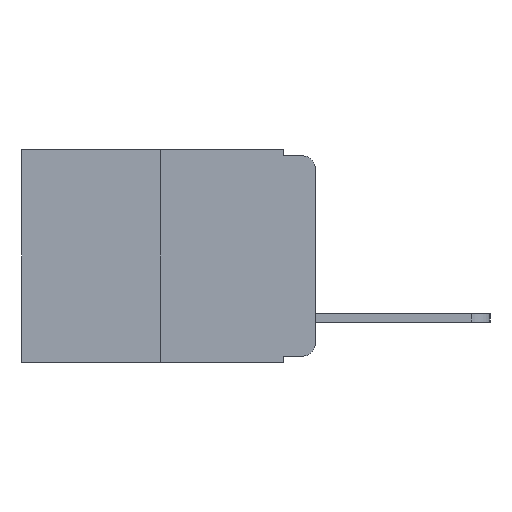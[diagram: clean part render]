
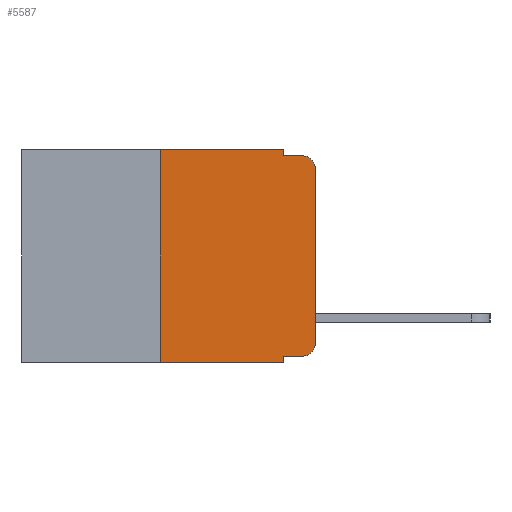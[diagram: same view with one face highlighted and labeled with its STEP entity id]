
A CAD part, left-side view. The second image highlights one B-rep face of the part: STEP entity #5587.
In plain terms, the highlighted planar face has unit normal (-1, 0, 0).
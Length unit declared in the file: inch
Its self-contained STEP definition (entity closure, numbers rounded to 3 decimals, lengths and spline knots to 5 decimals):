
#275 = VERTEX_POINT ( 'NONE', #3671 ) ;
#332 = VERTEX_POINT ( 'NONE', #5225 ) ;
#398 = AXIS2_PLACEMENT_3D ( 'NONE', #10428, #5423, #5416 ) ;
#938 = CARTESIAN_POINT ( 'NONE',  ( 0., 0.25, 0. ) ) ;
#1003 = DIRECTION ( 'NONE',  ( -1., 0., 0. ) ) ;
#1064 = DIRECTION ( 'NONE',  ( -1., 0., 0. ) ) ;
#1121 = DIRECTION ( 'NONE',  ( 0., 0., -1. ) ) ;
#1155 = VERTEX_POINT ( 'NONE', #1823 ) ;
#1223 = VERTEX_POINT ( 'NONE', #1884 ) ;
#1278 = DIRECTION ( 'NONE',  ( 0., 0., 1. ) ) ;
#1470 = CARTESIAN_POINT ( 'NONE',  ( 0., 0.25, 0. ) ) ;
#1720 = EDGE_CURVE ( 'NONE', #7638, #2436, #1954, .T. ) ;
#1823 = CARTESIAN_POINT ( 'NONE',  ( 0., 0.02, -0.01 ) ) ;
#1848 = EDGE_CURVE ( 'NONE', #1223, #10946, #10896, .T. ) ;
#1884 = CARTESIAN_POINT ( 'NONE',  ( 0., 0., -0.313 ) ) ;
#1954 = LINE ( 'NONE', #11174, #9098 ) ;
#2143 = LINE ( 'NONE', #1470, #2428 ) ;
#2428 = VECTOR ( 'NONE', #1278, 39.37008 ) ;
#2436 = VERTEX_POINT ( 'NONE', #6004 ) ;
#2580 = CIRCLE ( 'NONE', #11816, 0.02 ) ;
#2710 = EDGE_CURVE ( 'NONE', #8358, #332, #7228, .T. ) ;
#3127 = VERTEX_POINT ( 'NONE', #7342 ) ;
#3671 = CARTESIAN_POINT ( 'NONE',  ( 0., 0.051, -0.01 ) ) ;
#3939 = CIRCLE ( 'NONE', #5981, 0.02 ) ;
#4093 = EDGE_CURVE ( 'NONE', #3127, #8628, #4499, .T. ) ;
#4331 = LINE ( 'NONE', #4893, #11268 ) ;
#4339 = VECTOR ( 'NONE', #1121, 39.37008 ) ;
#4391 = VECTOR ( 'NONE', #6824, 39.37008 ) ;
#4499 = LINE ( 'NONE', #6081, #11632 ) ;
#4658 = EDGE_CURVE ( 'NONE', #8358, #8628, #6889, .T. ) ;
#4893 = CARTESIAN_POINT ( 'NONE',  ( 0., 0.051, 0. ) ) ;
#5225 = CARTESIAN_POINT ( 'NONE',  ( 0., 0.02, -0.333 ) ) ;
#5416 = DIRECTION ( 'NONE',  ( 0., 0., -1. ) ) ;
#5423 = DIRECTION ( 'NONE',  ( 1., 0., 0. ) ) ;
#5587 = ADVANCED_FACE ( 'NONE', ( #11594 ), #10465, .F. ) ;
#5734 = CARTESIAN_POINT ( 'NONE',  ( 0., 0.051, -0.333 ) ) ;
#5859 = DIRECTION ( 'NONE',  ( 0., 0., -1. ) ) ;
#5981 = AXIS2_PLACEMENT_3D ( 'NONE', #6794, #1003, #7716 ) ;
#6004 = CARTESIAN_POINT ( 'NONE',  ( 0., 0.051, 0. ) ) ;
#6037 = CARTESIAN_POINT ( 'NONE',  ( 0., 0., -0.03 ) ) ;
#6081 = CARTESIAN_POINT ( 'NONE',  ( 0., 0.473, -0.343 ) ) ;
#6360 = ORIENTED_EDGE ( 'NONE', *, *, #1848, .T. ) ;
#6423 = DIRECTION ( 'NONE',  ( 0., -1., 0. ) ) ;
#6488 = ORIENTED_EDGE ( 'NONE', *, *, #11796, .T. ) ;
#6523 = ORIENTED_EDGE ( 'NONE', *, *, #9559, .F. ) ;
#6599 = ORIENTED_EDGE ( 'NONE', *, *, #8447, .F. ) ;
#6634 = ORIENTED_EDGE ( 'NONE', *, *, #1720, .F. ) ;
#6703 = DIRECTION ( 'NONE',  ( 0., -1., 0. ) ) ;
#6794 = CARTESIAN_POINT ( 'NONE',  ( 0., 0.02, -0.313 ) ) ;
#6824 = DIRECTION ( 'NONE',  ( 0., -1., 0. ) ) ;
#6850 = CARTESIAN_POINT ( 'NONE',  ( 0., 0.02, -0.03 ) ) ;
#6889 = LINE ( 'NONE', #7921, #4339 ) ;
#6997 = VECTOR ( 'NONE', #6423, 39.37008 ) ;
#7017 = ORIENTED_EDGE ( 'NONE', *, *, #7216, .F. ) ;
#7019 = CARTESIAN_POINT ( 'NONE',  ( 0., 0.051, -0.343 ) ) ;
#7084 = ORIENTED_EDGE ( 'NONE', *, *, #4093, .T. ) ;
#7216 = EDGE_CURVE ( 'NONE', #3127, #7638, #2143, .T. ) ;
#7228 = LINE ( 'NONE', #9314, #4391 ) ;
#7263 = ORIENTED_EDGE ( 'NONE', *, *, #4658, .F. ) ;
#7295 = ORIENTED_EDGE ( 'NONE', *, *, #2710, .T. ) ;
#7329 = CARTESIAN_POINT ( 'NONE',  ( 0., 0.051, -0.01 ) ) ;
#7342 = CARTESIAN_POINT ( 'NONE',  ( 0., 0.25, -0.343 ) ) ;
#7431 = EDGE_LOOP ( 'NONE', ( #6360, #6488, #6523, #6599, #6634, #7017, #7084, #7263, #7295, #7758 ) ) ;
#7638 = VERTEX_POINT ( 'NONE', #938 ) ;
#7716 = DIRECTION ( 'NONE',  ( 0., 0., -1. ) ) ;
#7758 = ORIENTED_EDGE ( 'NONE', *, *, #11493, .T. ) ;
#7765 = DIRECTION ( 'NONE',  ( 0., 0., -1. ) ) ;
#7921 = CARTESIAN_POINT ( 'NONE',  ( 0., 0.051, 0. ) ) ;
#8331 = VECTOR ( 'NONE', #9049, 39.37008 ) ;
#8358 = VERTEX_POINT ( 'NONE', #5734 ) ;
#8447 = EDGE_CURVE ( 'NONE', #2436, #275, #4331, .T. ) ;
#8628 = VERTEX_POINT ( 'NONE', #7019 ) ;
#9049 = DIRECTION ( 'NONE',  ( 0., 0., 1. ) ) ;
#9098 = VECTOR ( 'NONE', #10126, 39.37008 ) ;
#9314 = CARTESIAN_POINT ( 'NONE',  ( 0., 0.051, -0.333 ) ) ;
#9324 = LINE ( 'NONE', #7329, #6997 ) ;
#9559 = EDGE_CURVE ( 'NONE', #275, #1155, #9324, .T. ) ;
#10126 = DIRECTION ( 'NONE',  ( 0., -1., 0. ) ) ;
#10428 = CARTESIAN_POINT ( 'NONE',  ( 0., 0.473, 0. ) ) ;
#10465 = PLANE ( 'NONE',  #398 ) ;
#10896 = LINE ( 'NONE', #12001, #8331 ) ;
#10946 = VERTEX_POINT ( 'NONE', #6037 ) ;
#11174 = CARTESIAN_POINT ( 'NONE',  ( 0., 0.473, 0. ) ) ;
#11268 = VECTOR ( 'NONE', #5859, 39.37008 ) ;
#11493 = EDGE_CURVE ( 'NONE', #332, #1223, #3939, .T. ) ;
#11594 = FACE_OUTER_BOUND ( 'NONE', #7431, .T. ) ;
#11632 = VECTOR ( 'NONE', #6703, 39.37008 ) ;
#11796 = EDGE_CURVE ( 'NONE', #10946, #1155, #2580, .T. ) ;
#11816 = AXIS2_PLACEMENT_3D ( 'NONE', #6850, #1064, #7765 ) ;
#12001 = CARTESIAN_POINT ( 'NONE',  ( 0., 0., 0. ) ) ;
